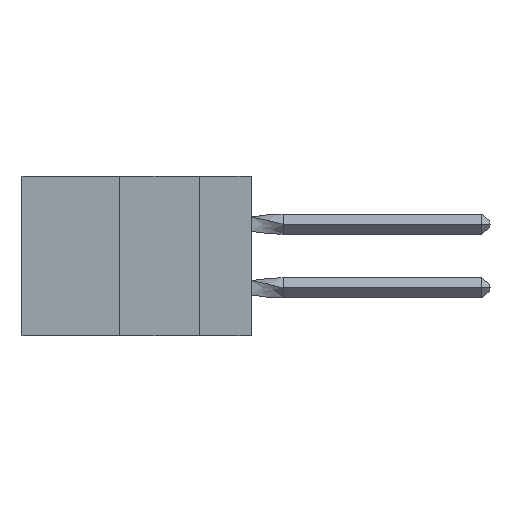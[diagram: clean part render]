
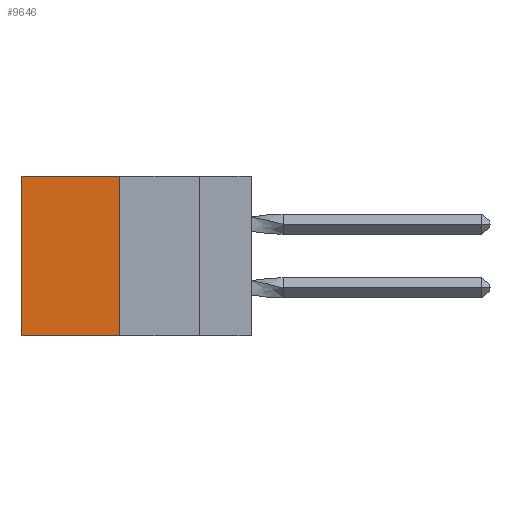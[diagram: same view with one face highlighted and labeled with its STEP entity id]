
A CAD part, left-side view. The second image highlights one B-rep face of the part: STEP entity #9646.
In plain terms, the highlighted planar face has unit normal (-1, 0, 0).
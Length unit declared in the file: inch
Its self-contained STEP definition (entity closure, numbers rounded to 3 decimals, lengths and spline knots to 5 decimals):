
#1322 = VERTEX_POINT ( 'NONE', #2140 ) ;
#1334 = FACE_OUTER_BOUND ( 'NONE', #11157, .T. ) ;
#1947 = CARTESIAN_POINT ( 'NONE',  ( 0.305, 0.413, 0. ) ) ;
#2140 = CARTESIAN_POINT ( 'NONE',  ( 0.305, 0.413, -0.5 ) ) ;
#2147 = VERTEX_POINT ( 'NONE', #7709 ) ;
#2458 = VERTEX_POINT ( 'NONE', #12482 ) ;
#2522 = DIRECTION ( 'NONE',  ( 0., 0., -1. ) ) ;
#3021 = CARTESIAN_POINT ( 'NONE',  ( 0.305, 0.413, -0.5 ) ) ;
#3993 = ORIENTED_EDGE ( 'NONE', *, *, #13258, .T. ) ;
#5386 = EDGE_CURVE ( 'NONE', #1322, #12079, #6335, .T. ) ;
#6335 = LINE ( 'NONE', #15244, #7129 ) ;
#6354 = ORIENTED_EDGE ( 'NONE', *, *, #9009, .F. ) ;
#7129 = VECTOR ( 'NONE', #12548, 39.37008 ) ;
#7574 = VECTOR ( 'NONE', #14522, 39.37008 ) ;
#7688 = DIRECTION ( 'NONE',  ( 0., 0., -1. ) ) ;
#7709 = CARTESIAN_POINT ( 'NONE',  ( 0.305, 0.413, 0. ) ) ;
#7737 = AXIS2_PLACEMENT_3D ( 'NONE', #3021, #14215, #8288 ) ;
#7774 = EDGE_CURVE ( 'NONE', #2458, #12079, #10695, .T. ) ;
#8098 = VECTOR ( 'NONE', #7688, 39.37008 ) ;
#8288 = DIRECTION ( 'NONE',  ( 0., 0., -1. ) ) ;
#8756 = LINE ( 'NONE', #1947, #7574 ) ;
#9009 = EDGE_CURVE ( 'NONE', #2147, #1322, #16305, .T. ) ;
#9646 = ADVANCED_FACE ( 'NONE', ( #1334 ), #10612, .F. ) ;
#9892 = VECTOR ( 'NONE', #2522, 39.37008 ) ;
#10612 = PLANE ( 'NONE',  #7737 ) ;
#10695 = LINE ( 'NONE', #11466, #9892 ) ;
#11088 = CARTESIAN_POINT ( 'NONE',  ( 0.305, 0.72, -0.5 ) ) ;
#11157 = EDGE_LOOP ( 'NONE', ( #11932, #14526, #6354, #3993 ) ) ;
#11466 = CARTESIAN_POINT ( 'NONE',  ( 0.305, 0.72, -0.5 ) ) ;
#11932 = ORIENTED_EDGE ( 'NONE', *, *, #7774, .T. ) ;
#12079 = VERTEX_POINT ( 'NONE', #11088 ) ;
#12482 = CARTESIAN_POINT ( 'NONE',  ( 0.305, 0.72, 0. ) ) ;
#12548 = DIRECTION ( 'NONE',  ( 0., 1., 0. ) ) ;
#13258 = EDGE_CURVE ( 'NONE', #2147, #2458, #8756, .T. ) ;
#14215 = DIRECTION ( 'NONE',  ( 1., 0., 0. ) ) ;
#14522 = DIRECTION ( 'NONE',  ( 0., 1., 0. ) ) ;
#14526 = ORIENTED_EDGE ( 'NONE', *, *, #5386, .F. ) ;
#15244 = CARTESIAN_POINT ( 'NONE',  ( 0.305, 0.413, -0.5 ) ) ;
#15296 = CARTESIAN_POINT ( 'NONE',  ( 0.305, 0.413, -0.5 ) ) ;
#16305 = LINE ( 'NONE', #15296, #8098 ) ;
